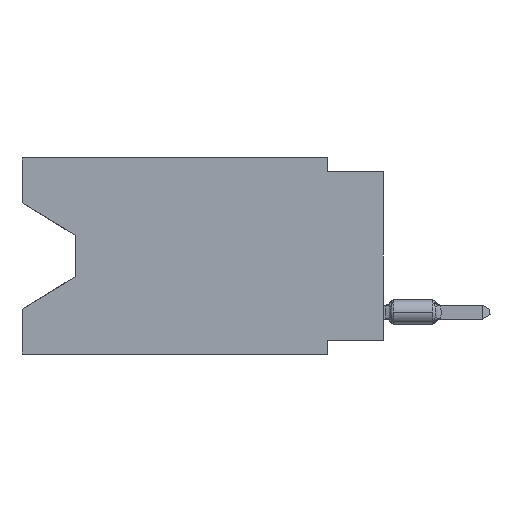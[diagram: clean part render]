
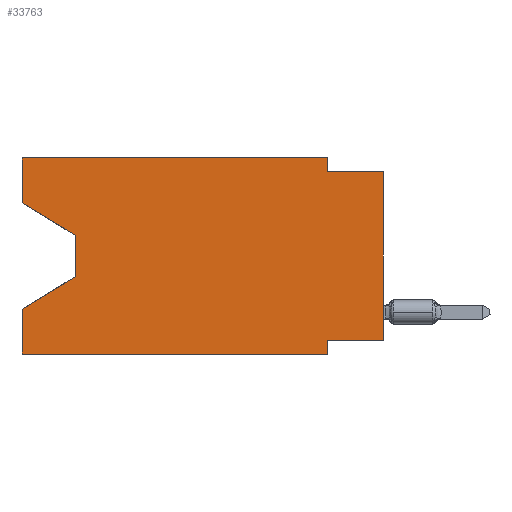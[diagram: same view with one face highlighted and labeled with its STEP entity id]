
A CAD part, left-side view. The second image highlights one B-rep face of the part: STEP entity #33763.
In plain terms, the highlighted planar face has unit normal (-1, 0, 0).
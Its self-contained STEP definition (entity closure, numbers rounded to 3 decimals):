
#45 = CARTESIAN_POINT ( 'NONE',  ( 0., 0., -8.255 ) ) ;
#148 = CARTESIAN_POINT ( 'NONE',  ( 0., 2.54, 0. ) ) ;
#808 = EDGE_CURVE ( 'NONE', #4149, #43943, #60944, .T. ) ;
#1121 = LINE ( 'NONE', #10771, #42488 ) ;
#1240 = VERTEX_POINT ( 'NONE', #43460 ) ;
#1963 = EDGE_CURVE ( 'NONE', #29075, #25445, #18568, .T. ) ;
#2045 = FACE_OUTER_BOUND ( 'NONE', #39868, .T. ) ;
#3604 = CARTESIAN_POINT ( 'NONE',  ( 0., 16.383, -6.852 ) ) ;
#3707 = VERTEX_POINT ( 'NONE', #14264 ) ;
#3758 = LINE ( 'NONE', #41917, #14413 ) ;
#4149 = VERTEX_POINT ( 'NONE', #148 ) ;
#4193 = VERTEX_POINT ( 'NONE', #33298 ) ;
#4230 = EDGE_CURVE ( 'NONE', #9751, #54673, #30743, .T. ) ;
#5307 = DIRECTION ( 'NONE',  ( 0., -1., 0. ) ) ;
#5328 = VERTEX_POINT ( 'NONE', #45 ) ;
#5718 = EDGE_CURVE ( 'NONE', #43943, #4193, #41246, .T. ) ;
#6045 = DIRECTION ( 'NONE',  ( 0., 0.855, -0.519 ) ) ;
#7693 = DIRECTION ( 'NONE',  ( 0., 0., -1. ) ) ;
#8408 = CARTESIAN_POINT ( 'NONE',  ( 0., 2.54, 0. ) ) ;
#9691 = EDGE_CURVE ( 'NONE', #1240, #30624, #41466, .T. ) ;
#9751 = VERTEX_POINT ( 'NONE', #14550 ) ;
#10771 = CARTESIAN_POINT ( 'NONE',  ( 0., 16.383, 0. ) ) ;
#11940 = CARTESIAN_POINT ( 'NONE',  ( 0., 13.97, -5.385 ) ) ;
#12057 = EDGE_CURVE ( 'NONE', #5328, #1240, #18709, .T. ) ;
#12166 = LINE ( 'NONE', #50309, #19130 ) ;
#14031 = CARTESIAN_POINT ( 'NONE',  ( 0., 0., -8.255 ) ) ;
#14264 = CARTESIAN_POINT ( 'NONE',  ( 0., 16.383, 0. ) ) ;
#14413 = VECTOR ( 'NONE', #37232, 1000. ) ;
#14550 = CARTESIAN_POINT ( 'NONE',  ( 0., 13.97, -5.385 ) ) ;
#14915 = EDGE_CURVE ( 'NONE', #37669, #30624, #49353, .T. ) ;
#15378 = LINE ( 'NONE', #25090, #23564 ) ;
#15679 = DIRECTION ( 'NONE',  ( 0., 0., 1. ) ) ;
#16108 = DIRECTION ( 'NONE',  ( 0., 0., -1. ) ) ;
#18145 = ORIENTED_EDGE ( 'NONE', *, *, #4230, .T. ) ;
#18568 = LINE ( 'NONE', #37971, #47591 ) ;
#18709 = LINE ( 'NONE', #14031, #30489 ) ;
#18819 = VECTOR ( 'NONE', #6045, 1000. ) ;
#19130 = VECTOR ( 'NONE', #45611, 1000. ) ;
#19330 = ORIENTED_EDGE ( 'NONE', *, *, #1963, .T. ) ;
#20355 = ORIENTED_EDGE ( 'NONE', *, *, #808, .F. ) ;
#20962 = ORIENTED_EDGE ( 'NONE', *, *, #9691, .F. ) ;
#22227 = ORIENTED_EDGE ( 'NONE', *, *, #49863, .F. ) ;
#22458 = CARTESIAN_POINT ( 'NONE',  ( 0., 13.97, -3.505 ) ) ;
#22653 = DIRECTION ( 'NONE',  ( 0., -0.855, -0.519 ) ) ;
#23036 = CARTESIAN_POINT ( 'NONE',  ( 0., 2.54, -8.89 ) ) ;
#23082 = DIRECTION ( 'NONE',  ( 0., 0., -1. ) ) ;
#23109 = DIRECTION ( 'NONE',  ( 0., -1., 0. ) ) ;
#23171 = CARTESIAN_POINT ( 'NONE',  ( 0., 2.54, -8.89 ) ) ;
#23564 = VECTOR ( 'NONE', #15679, 1000. ) ;
#25090 = CARTESIAN_POINT ( 'NONE',  ( 0., 0., 0. ) ) ;
#25445 = VERTEX_POINT ( 'NONE', #53278 ) ;
#25916 = EDGE_CURVE ( 'NONE', #5328, #4193, #15378, .T. ) ;
#27224 = ORIENTED_EDGE ( 'NONE', *, *, #36781, .F. ) ;
#29075 = VERTEX_POINT ( 'NONE', #31783 ) ;
#29948 = VECTOR ( 'NONE', #23109, 1000. ) ;
#30024 = CARTESIAN_POINT ( 'NONE',  ( 0., 16.383, -8.89 ) ) ;
#30489 = VECTOR ( 'NONE', #33127, 1000. ) ;
#30624 = VERTEX_POINT ( 'NONE', #23171 ) ;
#30743 = LINE ( 'NONE', #11940, #18819 ) ;
#30816 = PLANE ( 'NONE',  #31035 ) ;
#31035 = AXIS2_PLACEMENT_3D ( 'NONE', #35498, #48622, #16108 ) ;
#31533 = ORIENTED_EDGE ( 'NONE', *, *, #25916, .T. ) ;
#31733 = CARTESIAN_POINT ( 'NONE',  ( 0., 16.383, -8.89 ) ) ;
#31783 = CARTESIAN_POINT ( 'NONE',  ( 0., 16.383, -2.038 ) ) ;
#31839 = LINE ( 'NONE', #22458, #42121 ) ;
#32387 = ORIENTED_EDGE ( 'NONE', *, *, #5718, .F. ) ;
#33127 = DIRECTION ( 'NONE',  ( 0., 1., 0. ) ) ;
#33298 = CARTESIAN_POINT ( 'NONE',  ( 0., 0., -0.635 ) ) ;
#33763 = ADVANCED_FACE ( 'NONE', ( #2045 ), #30816, .F. ) ;
#35237 = ORIENTED_EDGE ( 'NONE', *, *, #14915, .T. ) ;
#35498 = CARTESIAN_POINT ( 'NONE',  ( 0., 16.383, 0. ) ) ;
#36781 = EDGE_CURVE ( 'NONE', #3707, #4149, #12166, .T. ) ;
#37232 = DIRECTION ( 'NONE',  ( 0., 0., 1. ) ) ;
#37669 = VERTEX_POINT ( 'NONE', #31733 ) ;
#37971 = CARTESIAN_POINT ( 'NONE',  ( 0., 16.383, -2.038 ) ) ;
#39241 = EDGE_CURVE ( 'NONE', #25445, #9751, #31839, .T. ) ;
#39868 = EDGE_LOOP ( 'NONE', ( #19330, #44165, #18145, #22227, #35237, #20962, #40091, #31533, #32387, #20355, #27224, #58604 ) ) ;
#40091 = ORIENTED_EDGE ( 'NONE', *, *, #12057, .F. ) ;
#41246 = LINE ( 'NONE', #60298, #29948 ) ;
#41466 = LINE ( 'NONE', #23036, #60277 ) ;
#41485 = VECTOR ( 'NONE', #5307, 1000. ) ;
#41917 = CARTESIAN_POINT ( 'NONE',  ( 0., 16.383, 0. ) ) ;
#42121 = VECTOR ( 'NONE', #23082, 1000. ) ;
#42488 = VECTOR ( 'NONE', #49237, 1000. ) ;
#43460 = CARTESIAN_POINT ( 'NONE',  ( 0., 2.54, -8.255 ) ) ;
#43943 = VERTEX_POINT ( 'NONE', #47817 ) ;
#44165 = ORIENTED_EDGE ( 'NONE', *, *, #39241, .T. ) ;
#45611 = DIRECTION ( 'NONE',  ( 0., -1., 0. ) ) ;
#47591 = VECTOR ( 'NONE', #22653, 1000. ) ;
#47817 = CARTESIAN_POINT ( 'NONE',  ( 0., 2.54, -0.635 ) ) ;
#48622 = DIRECTION ( 'NONE',  ( 1., 0., 0. ) ) ;
#49237 = DIRECTION ( 'NONE',  ( 0., 0., 1. ) ) ;
#49353 = LINE ( 'NONE', #30024, #41485 ) ;
#49863 = EDGE_CURVE ( 'NONE', #37669, #54673, #3758, .T. ) ;
#50309 = CARTESIAN_POINT ( 'NONE',  ( 0., 16.383, 0. ) ) ;
#50477 = EDGE_CURVE ( 'NONE', #29075, #3707, #1121, .T. ) ;
#53278 = CARTESIAN_POINT ( 'NONE',  ( 0., 13.97, -3.505 ) ) ;
#54673 = VERTEX_POINT ( 'NONE', #3604 ) ;
#55452 = VECTOR ( 'NONE', #60626, 1000. ) ;
#58604 = ORIENTED_EDGE ( 'NONE', *, *, #50477, .F. ) ;
#60277 = VECTOR ( 'NONE', #7693, 1000. ) ;
#60298 = CARTESIAN_POINT ( 'NONE',  ( 0., 0., -0.635 ) ) ;
#60626 = DIRECTION ( 'NONE',  ( 0., 0., -1. ) ) ;
#60944 = LINE ( 'NONE', #8408, #55452 ) ;
